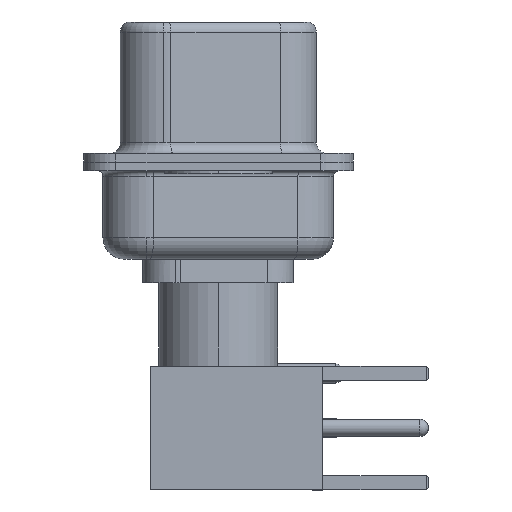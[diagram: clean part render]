
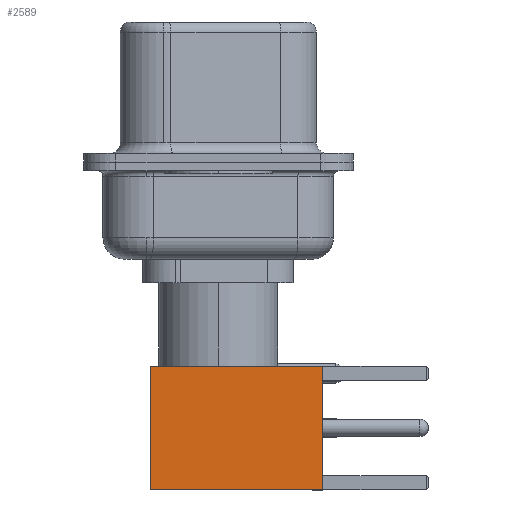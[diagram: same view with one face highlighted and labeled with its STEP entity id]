
A CAD part, left-side view. The second image highlights one B-rep face of the part: STEP entity #2589.
In plain terms, the highlighted face is planar.
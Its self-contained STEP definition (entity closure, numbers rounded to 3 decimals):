
#1553 = VERTEX_POINT ( 'NONE', #12805 ) ;
#2090 = VECTOR ( 'NONE', #2123, 1000. ) ;
#2123 = DIRECTION ( 'NONE',  ( 0., 0., -1. ) ) ;
#2397 = VECTOR ( 'NONE', #11392, 1000. ) ;
#2562 = ORIENTED_EDGE ( 'NONE', *, *, #23281, .F. ) ;
#2589 = ADVANCED_FACE ( 'NONE', ( #13114 ), #11437, .T. ) ;
#3297 = VERTEX_POINT ( 'NONE', #12224 ) ;
#4293 = LINE ( 'NONE', #7596, #14894 ) ;
#4715 = CARTESIAN_POINT ( 'NONE',  ( 0., 2.875, 8. ) ) ;
#7596 = CARTESIAN_POINT ( 'NONE',  ( 0., 2.875, 0. ) ) ;
#7881 = VERTEX_POINT ( 'NONE', #8695 ) ;
#8245 = VECTOR ( 'NONE', #19436, 1000. ) ;
#8693 = EDGE_CURVE ( 'NONE', #20473, #1553, #10267, .T. ) ;
#8695 = CARTESIAN_POINT ( 'NONE',  ( -2.875, 2.875, 0. ) ) ;
#10267 = LINE ( 'NONE', #4715, #2397 ) ;
#11392 = DIRECTION ( 'NONE',  ( -1., 0., 0. ) ) ;
#11437 = PLANE ( 'NONE',  #11573 ) ;
#11573 = AXIS2_PLACEMENT_3D ( 'NONE', #15129, #13471, #16763 ) ;
#11699 = EDGE_LOOP ( 'NONE', ( #12399, #16301, #2562, #18575 ) ) ;
#11864 = LINE ( 'NONE', #22876, #8245 ) ;
#12224 = CARTESIAN_POINT ( 'NONE',  ( 2.875, 2.875, 0. ) ) ;
#12399 = ORIENTED_EDGE ( 'NONE', *, *, #17389, .T. ) ;
#12557 = LINE ( 'NONE', #17988, #2090 ) ;
#12805 = CARTESIAN_POINT ( 'NONE',  ( -2.875, 2.875, 8. ) ) ;
#13114 = FACE_OUTER_BOUND ( 'NONE', #11699, .T. ) ;
#13180 = DIRECTION ( 'NONE',  ( -1., 0., 0. ) ) ;
#13471 = DIRECTION ( 'NONE',  ( 0., 1., 0. ) ) ;
#13942 = CARTESIAN_POINT ( 'NONE',  ( 2.875, 2.875, 8. ) ) ;
#14894 = VECTOR ( 'NONE', #13180, 1000. ) ;
#15079 = EDGE_CURVE ( 'NONE', #3297, #7881, #4293, .T. ) ;
#15129 = CARTESIAN_POINT ( 'NONE',  ( 2.875, 2.875, 0. ) ) ;
#16301 = ORIENTED_EDGE ( 'NONE', *, *, #15079, .T. ) ;
#16763 = DIRECTION ( 'NONE',  ( 0., 0., 1. ) ) ;
#17389 = EDGE_CURVE ( 'NONE', #20473, #3297, #11864, .T. ) ;
#17988 = CARTESIAN_POINT ( 'NONE',  ( -2.875, 2.875, 0. ) ) ;
#18575 = ORIENTED_EDGE ( 'NONE', *, *, #8693, .F. ) ;
#19436 = DIRECTION ( 'NONE',  ( 0., 0., -1. ) ) ;
#20473 = VERTEX_POINT ( 'NONE', #13942 ) ;
#22876 = CARTESIAN_POINT ( 'NONE',  ( 2.875, 2.875, 0. ) ) ;
#23281 = EDGE_CURVE ( 'NONE', #1553, #7881, #12557, .T. ) ;
